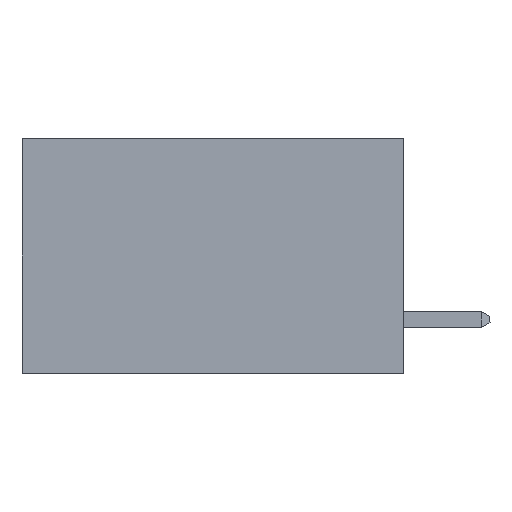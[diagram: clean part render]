
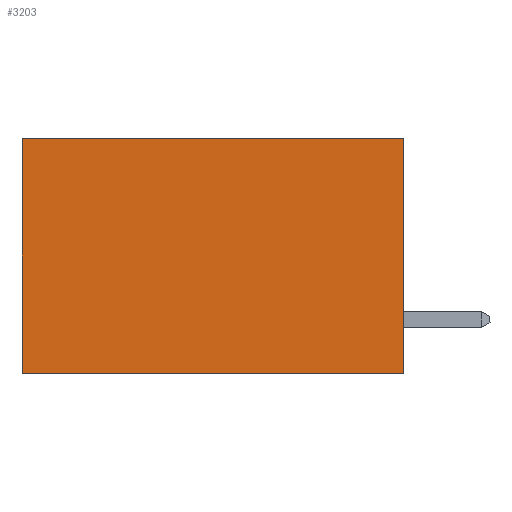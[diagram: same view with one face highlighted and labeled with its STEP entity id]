
A CAD part, left-side view. The second image highlights one B-rep face of the part: STEP entity #3203.
In plain terms, the highlighted planar face has unit normal (-1, 0, 0).
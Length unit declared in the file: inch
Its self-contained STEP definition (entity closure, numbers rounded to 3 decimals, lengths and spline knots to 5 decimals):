
#831 = CARTESIAN_POINT ( 'NONE',  ( 0.2875, 0.6, 0. ) ) ;
#1073 = DIRECTION ( 'NONE',  ( 0., 1., 0. ) ) ;
#1384 = CARTESIAN_POINT ( 'NONE',  ( 0.2875, 0., -0.37 ) ) ;
#2223 = VERTEX_POINT ( 'NONE', #23322 ) ;
#2561 = ORIENTED_EDGE ( 'NONE', *, *, #18179, .F. ) ;
#3203 = ADVANCED_FACE ( 'NONE', ( #5246 ), #9649, .F. ) ;
#4653 = EDGE_CURVE ( 'NONE', #16911, #6175, #20462, .T. ) ;
#4795 = EDGE_CURVE ( 'NONE', #12790, #6175, #10189, .T. ) ;
#5100 = CARTESIAN_POINT ( 'NONE',  ( 0.2875, 0., 0. ) ) ;
#5246 = FACE_OUTER_BOUND ( 'NONE', #13794, .T. ) ;
#6175 = VERTEX_POINT ( 'NONE', #13472 ) ;
#7013 = EDGE_CURVE ( 'NONE', #2223, #12790, #19982, .T. ) ;
#9584 = DIRECTION ( 'NONE',  ( 1., 0., 0. ) ) ;
#9638 = CARTESIAN_POINT ( 'NONE',  ( 0.2875, 0., 0. ) ) ;
#9643 = DIRECTION ( 'NONE',  ( 0., 0., -1. ) ) ;
#9649 = PLANE ( 'NONE',  #11234 ) ;
#9712 = CARTESIAN_POINT ( 'NONE',  ( 0.2875, 0., 0. ) ) ;
#10189 = LINE ( 'NONE', #23249, #22246 ) ;
#11234 = AXIS2_PLACEMENT_3D ( 'NONE', #9712, #9584, #9643 ) ;
#12601 = ORIENTED_EDGE ( 'NONE', *, *, #4795, .T. ) ;
#12790 = VERTEX_POINT ( 'NONE', #831 ) ;
#13231 = VECTOR ( 'NONE', #16499, 39.37008 ) ;
#13472 = CARTESIAN_POINT ( 'NONE',  ( 0.2875, 0.6, -0.37 ) ) ;
#13794 = EDGE_LOOP ( 'NONE', ( #12601, #24694, #2561, #26825 ) ) ;
#16499 = DIRECTION ( 'NONE',  ( 0., 1., 0. ) ) ;
#16911 = VERTEX_POINT ( 'NONE', #24969 ) ;
#18179 = EDGE_CURVE ( 'NONE', #2223, #16911, #26252, .T. ) ;
#19982 = LINE ( 'NONE', #9638, #13231 ) ;
#20239 = VECTOR ( 'NONE', #27802, 39.37008 ) ;
#20462 = LINE ( 'NONE', #1384, #25084 ) ;
#22246 = VECTOR ( 'NONE', #23216, 39.37008 ) ;
#23216 = DIRECTION ( 'NONE',  ( 0., 0., -1. ) ) ;
#23249 = CARTESIAN_POINT ( 'NONE',  ( 0.2875, 0.6, 0. ) ) ;
#23322 = CARTESIAN_POINT ( 'NONE',  ( 0.2875, 0., 0. ) ) ;
#24694 = ORIENTED_EDGE ( 'NONE', *, *, #4653, .F. ) ;
#24969 = CARTESIAN_POINT ( 'NONE',  ( 0.2875, 0., -0.37 ) ) ;
#25084 = VECTOR ( 'NONE', #1073, 39.37008 ) ;
#26252 = LINE ( 'NONE', #5100, #20239 ) ;
#26825 = ORIENTED_EDGE ( 'NONE', *, *, #7013, .T. ) ;
#27802 = DIRECTION ( 'NONE',  ( 0., 0., -1. ) ) ;
